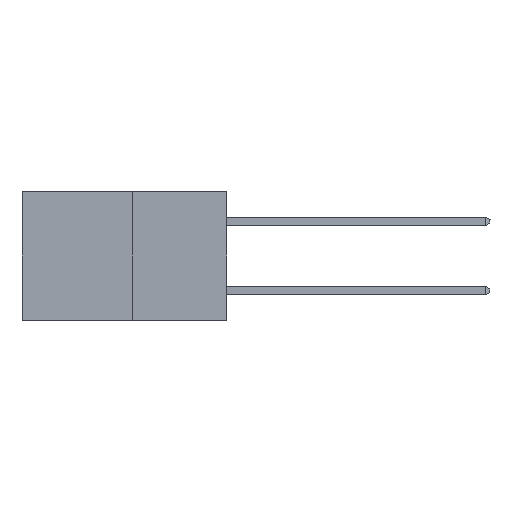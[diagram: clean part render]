
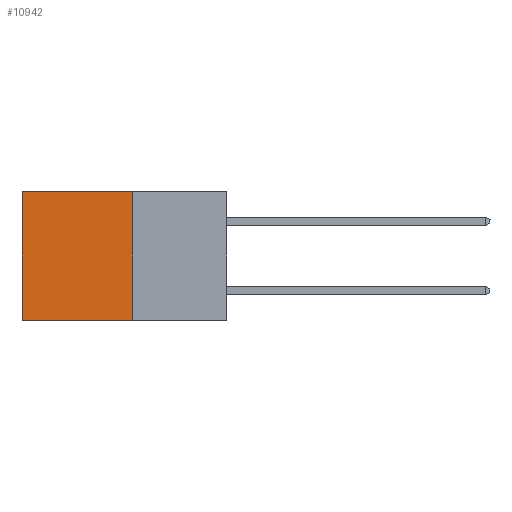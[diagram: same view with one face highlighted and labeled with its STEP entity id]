
A CAD part, left-side view. The second image highlights one B-rep face of the part: STEP entity #10942.
In plain terms, the highlighted planar face has unit normal (-1, 0, 0).
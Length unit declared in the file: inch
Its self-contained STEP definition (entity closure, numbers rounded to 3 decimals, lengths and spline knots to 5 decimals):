
#200 = CARTESIAN_POINT ( 'NONE',  ( 0.277, 0.27, 0. ) ) ;
#264 = VERTEX_POINT ( 'NONE', #5360 ) ;
#790 = EDGE_CURVE ( 'NONE', #11603, #9558, #10919, .T. ) ;
#1505 = CARTESIAN_POINT ( 'NONE',  ( 0.277, 0.27, 0. ) ) ;
#1576 = DIRECTION ( 'NONE',  ( 1., 0., 0. ) ) ;
#1885 = VECTOR ( 'NONE', #4990, 39.37008 ) ;
#1948 = DIRECTION ( 'NONE',  ( 0., 0., -1. ) ) ;
#2300 = VECTOR ( 'NONE', #12509, 39.37008 ) ;
#2653 = PLANE ( 'NONE',  #2751 ) ;
#2751 = AXIS2_PLACEMENT_3D ( 'NONE', #8231, #1576, #9302 ) ;
#3989 = CARTESIAN_POINT ( 'NONE',  ( 0.277, 0.27, -0.37 ) ) ;
#4585 = ORIENTED_EDGE ( 'NONE', *, *, #4715, .F. ) ;
#4675 = VECTOR ( 'NONE', #1948, 39.37008 ) ;
#4715 = EDGE_CURVE ( 'NONE', #9558, #264, #13476, .T. ) ;
#4990 = DIRECTION ( 'NONE',  ( 0., 0., -1. ) ) ;
#5360 = CARTESIAN_POINT ( 'NONE',  ( 0.277, 0.59, -0.37 ) ) ;
#7566 = EDGE_CURVE ( 'NONE', #9325, #264, #7988, .T. ) ;
#7690 = EDGE_CURVE ( 'NONE', #11603, #9325, #11253, .T. ) ;
#7988 = LINE ( 'NONE', #9078, #4675 ) ;
#8231 = CARTESIAN_POINT ( 'NONE',  ( 0.277, 0.27, -0.37 ) ) ;
#8458 = DIRECTION ( 'NONE',  ( 0., 1., 0. ) ) ;
#8815 = VECTOR ( 'NONE', #8458, 39.37008 ) ;
#8869 = CARTESIAN_POINT ( 'NONE',  ( 0.277, 0.27, -0.37 ) ) ;
#9074 = ORIENTED_EDGE ( 'NONE', *, *, #790, .F. ) ;
#9078 = CARTESIAN_POINT ( 'NONE',  ( 0.277, 0.59, -0.37 ) ) ;
#9302 = DIRECTION ( 'NONE',  ( 0., 0., -1. ) ) ;
#9325 = VERTEX_POINT ( 'NONE', #11371 ) ;
#9515 = EDGE_LOOP ( 'NONE', ( #12478, #4585, #9074, #11507 ) ) ;
#9558 = VERTEX_POINT ( 'NONE', #8869 ) ;
#10919 = LINE ( 'NONE', #3989, #1885 ) ;
#10942 = ADVANCED_FACE ( 'NONE', ( #11422 ), #2653, .F. ) ;
#11253 = LINE ( 'NONE', #200, #8815 ) ;
#11371 = CARTESIAN_POINT ( 'NONE',  ( 0.277, 0.59, 0. ) ) ;
#11422 = FACE_OUTER_BOUND ( 'NONE', #9515, .T. ) ;
#11507 = ORIENTED_EDGE ( 'NONE', *, *, #7690, .T. ) ;
#11603 = VERTEX_POINT ( 'NONE', #1505 ) ;
#12478 = ORIENTED_EDGE ( 'NONE', *, *, #7566, .T. ) ;
#12509 = DIRECTION ( 'NONE',  ( 0., 1., 0. ) ) ;
#12552 = CARTESIAN_POINT ( 'NONE',  ( 0.277, 0.27, -0.37 ) ) ;
#13476 = LINE ( 'NONE', #12552, #2300 ) ;
